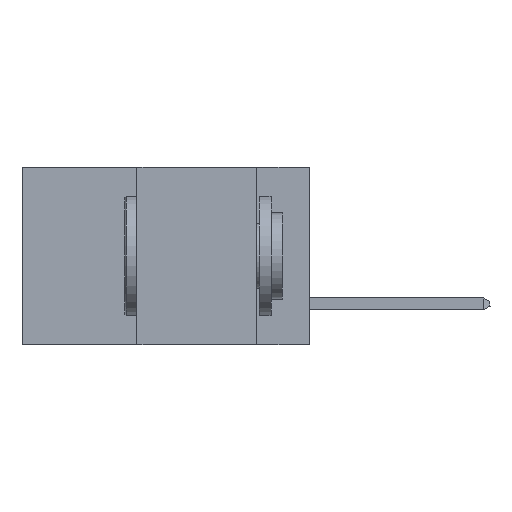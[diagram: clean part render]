
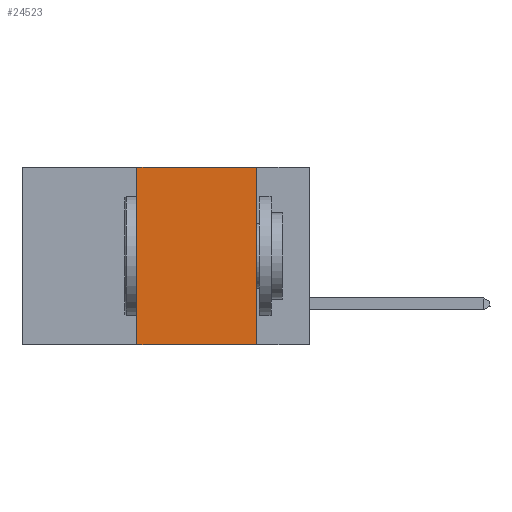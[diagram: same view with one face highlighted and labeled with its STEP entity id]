
A CAD part, left-side view. The second image highlights one B-rep face of the part: STEP entity #24523.
In plain terms, the highlighted planar face has unit normal (-1, 0, 0).
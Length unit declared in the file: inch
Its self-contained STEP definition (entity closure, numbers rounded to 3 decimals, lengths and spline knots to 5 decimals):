
#1220 = CARTESIAN_POINT ( 'NONE',  ( 0., 0.36, 0. ) ) ;
#2662 = EDGE_CURVE ( 'NONE', #13455, #13987, #3610, .T. ) ;
#2737 = EDGE_CURVE ( 'NONE', #25557, #30572, #41667, .T. ) ;
#3610 = LINE ( 'NONE', #35254, #13497 ) ;
#3668 = CARTESIAN_POINT ( 'NONE',  ( 0., 0.36, 0. ) ) ;
#4327 = ORIENTED_EDGE ( 'NONE', *, *, #15935, .F. ) ;
#5616 = EDGE_CURVE ( 'NONE', #25557, #13987, #32874, .T. ) ;
#6924 = CARTESIAN_POINT ( 'NONE',  ( 0., 0.11, 0. ) ) ;
#8601 = LINE ( 'NONE', #20510, #47274 ) ;
#9674 = DIRECTION ( 'NONE',  ( 0., 0., 1. ) ) ;
#10764 = VECTOR ( 'NONE', #45131, 39.37008 ) ;
#11836 = EDGE_LOOP ( 'NONE', ( #19401, #4327, #42439, #20716 ) ) ;
#13455 = VERTEX_POINT ( 'NONE', #6924 ) ;
#13497 = VECTOR ( 'NONE', #28594, 39.37008 ) ;
#13987 = VERTEX_POINT ( 'NONE', #38053 ) ;
#14120 = AXIS2_PLACEMENT_3D ( 'NONE', #35049, #46732, #27048 ) ;
#15935 = EDGE_CURVE ( 'NONE', #30572, #13455, #8601, .T. ) ;
#19401 = ORIENTED_EDGE ( 'NONE', *, *, #2662, .F. ) ;
#20510 = CARTESIAN_POINT ( 'NONE',  ( 0., 0.6, 0. ) ) ;
#20716 = ORIENTED_EDGE ( 'NONE', *, *, #5616, .T. ) ;
#24523 = ADVANCED_FACE ( 'NONE', ( #36089 ), #31112, .F. ) ;
#25557 = VERTEX_POINT ( 'NONE', #40097 ) ;
#25820 = VECTOR ( 'NONE', #9674, 39.37008 ) ;
#27048 = DIRECTION ( 'NONE',  ( 0., 0., -1. ) ) ;
#28594 = DIRECTION ( 'NONE',  ( 0., 0., -1. ) ) ;
#30572 = VERTEX_POINT ( 'NONE', #3668 ) ;
#31112 = PLANE ( 'NONE',  #14120 ) ;
#32785 = CARTESIAN_POINT ( 'NONE',  ( 0., 0.6, -0.37 ) ) ;
#32874 = LINE ( 'NONE', #32785, #10764 ) ;
#35049 = CARTESIAN_POINT ( 'NONE',  ( 0., 0.6, 0. ) ) ;
#35254 = CARTESIAN_POINT ( 'NONE',  ( 0., 0.11, 0. ) ) ;
#36089 = FACE_OUTER_BOUND ( 'NONE', #11836, .T. ) ;
#36393 = DIRECTION ( 'NONE',  ( 0., -1., 0. ) ) ;
#38053 = CARTESIAN_POINT ( 'NONE',  ( 0., 0.11, -0.37 ) ) ;
#40097 = CARTESIAN_POINT ( 'NONE',  ( 0., 0.36, -0.37 ) ) ;
#41667 = LINE ( 'NONE', #1220, #25820 ) ;
#42439 = ORIENTED_EDGE ( 'NONE', *, *, #2737, .F. ) ;
#45131 = DIRECTION ( 'NONE',  ( 0., -1., 0. ) ) ;
#46732 = DIRECTION ( 'NONE',  ( 1., 0., 0. ) ) ;
#47274 = VECTOR ( 'NONE', #36393, 39.37008 ) ;
